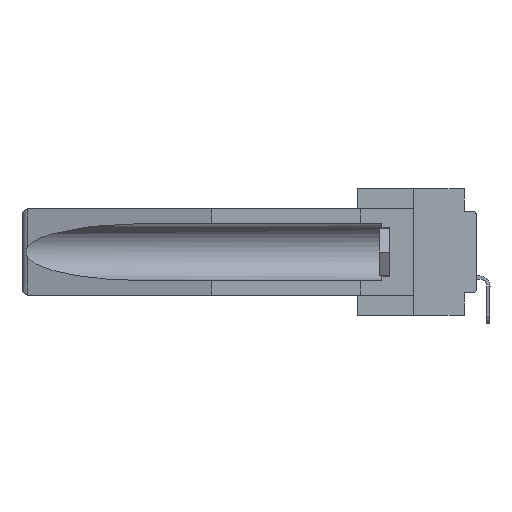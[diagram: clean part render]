
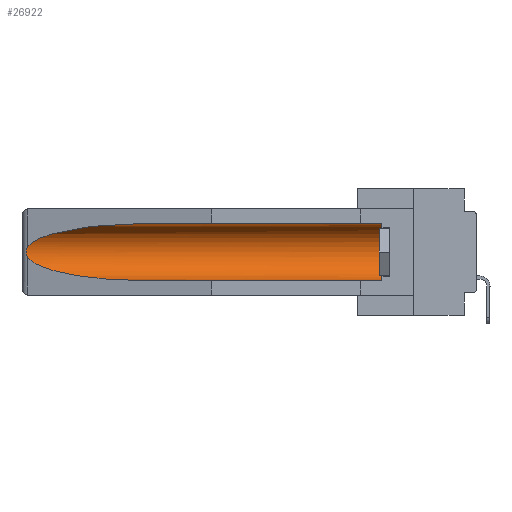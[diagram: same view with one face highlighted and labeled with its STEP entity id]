
A CAD part, left-side view. The second image highlights one B-rep face of the part: STEP entity #26922.
In plain terms, the highlighted cylindrical face has radius 2.857 mm (diameter 5.715 mm), a partial arc.
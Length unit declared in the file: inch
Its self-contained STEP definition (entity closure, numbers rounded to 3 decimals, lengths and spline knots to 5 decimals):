
#720 = DIRECTION ( 'NONE',  ( 0., 0., 1. ) ) ;
#1542 = EDGE_CURVE ( 'NONE', #3115, #8334, #3352, .T. ) ;
#2309 = ORIENTED_EDGE ( 'NONE', *, *, #4685, .T. ) ;
#2797 = EDGE_CURVE ( 'NONE', #3901, #11828, #21291, .T. ) ;
#2966 = CARTESIAN_POINT ( 'NONE',  ( 0.155, -0.30754, -0.1715 ) ) ;
#3114 = CARTESIAN_POINT ( 'NONE',  ( 0.2673, 1.5327, -0.16383 ) ) ;
#3115 = VERTEX_POINT ( 'NONE', #5909 ) ;
#3352 =( BOUNDED_CURVE ( )  B_SPLINE_CURVE ( 3, ( #6655, #21371, #31257, #21514 ),
 .UNSPECIFIED., .F., .T. ) 
 B_SPLINE_CURVE_WITH_KNOTS ( ( 4, 4 ),
 ( 4.71239, 6.08839 ),
 .UNSPECIFIED. ) 
 CURVE ( )  GEOMETRIC_REPRESENTATION_ITEM ( )  RATIONAL_B_SPLINE_CURVE ( ( 1., 0.848, 0.848, 1. ) ) 
 REPRESENTATION_ITEM ( '' )  );
#3901 = VERTEX_POINT ( 'NONE', #6263 ) ;
#4042 = ORIENTED_EDGE ( 'NONE', *, *, #2797, .F. ) ;
#4331 = CARTESIAN_POINT ( 'NONE',  ( 0.155, -0.30754, -0.284 ) ) ;
#4685 = EDGE_CURVE ( 'NONE', #8334, #18332, #13291, .T. ) ;
#4689 = VECTOR ( 'NONE', #21474, 39.37008 ) ;
#4727 = DIRECTION ( 'NONE',  ( 0., 0., 1. ) ) ;
#4944 = EDGE_CURVE ( 'NONE', #3901, #30158, #30249, .T. ) ;
#5623 = CARTESIAN_POINT ( 'NONE',  ( 0.155, 1.07973, -0.284 ) ) ;
#5909 = CARTESIAN_POINT ( 'NONE',  ( 0.155, 1.07973, -0.059 ) ) ;
#6025 = CARTESIAN_POINT ( 'NONE',  ( 0.2673, 1.53269, -0.17917 ) ) ;
#6038 = FACE_OUTER_BOUND ( 'NONE', #9230, .T. ) ;
#6116 = CARTESIAN_POINT ( 'NONE',  ( 0.21114, 1.30732, -0.284 ) ) ;
#6263 = CARTESIAN_POINT ( 'NONE',  ( 0.155, 0.126, -0.284 ) ) ;
#6655 = CARTESIAN_POINT ( 'NONE',  ( 0.155, 1.07973, -0.059 ) ) ;
#6661 = ORIENTED_EDGE ( 'NONE', *, *, #18236, .T. ) ;
#6783 = LINE ( 'NONE', #21328, #4689 ) ;
#8304 = CARTESIAN_POINT ( 'NONE',  ( 0.26655, 1.53094, -0.18657 ) ) ;
#8334 = VERTEX_POINT ( 'NONE', #29628 ) ;
#9230 = EDGE_LOOP ( 'NONE', ( #31022, #2309, #22160, #4042, #15883, #6661 ) ) ;
#10874 = CARTESIAN_POINT ( 'NONE',  ( 0.26597, 1.5296, -0.19026 ) ) ;
#11828 = VERTEX_POINT ( 'NONE', #5623 ) ;
#11921 = DIRECTION ( 'NONE',  ( 0., 1., 0. ) ) ;
#12840 = CARTESIAN_POINT ( 'NONE',  ( 0.26537, 1.52718, -0.14972 ) ) ;
#13243 = DIRECTION ( 'NONE',  ( 0., -1., 0. ) ) ;
#13280 =( BOUNDED_CURVE ( )  B_SPLINE_CURVE ( 3, ( #14213, #24045, #6116, #24677 ),
 .UNSPECIFIED., .F., .T. ) 
 B_SPLINE_CURVE_WITH_KNOTS ( ( 4, 4 ),
 ( 0.1948, 1.5708 ),
 .UNSPECIFIED. ) 
 CURVE ( )  GEOMETRIC_REPRESENTATION_ITEM ( )  RATIONAL_B_SPLINE_CURVE ( ( 1., 0.848, 0.848, 1. ) ) 
 REPRESENTATION_ITEM ( '' )  );
#13291 = B_SPLINE_CURVE_WITH_KNOTS ( 'NONE', 3,
 ( #12840, #20267, #30169, #3114, #28190, #20566, #6025, #8304, #10874, #18153 ),
 .UNSPECIFIED., .F., .F.,
 ( 4, 2, 2, 2, 4 ),
 ( 0., 0.00029, 0.00058, 0.00087, 0.00117 ),
 .UNSPECIFIED. ) ;
#13492 = DIRECTION ( 'NONE',  ( 0., 1., 0. ) ) ;
#14213 = CARTESIAN_POINT ( 'NONE',  ( 0.26537, 1.52718, -0.19328 ) ) ;
#15883 = ORIENTED_EDGE ( 'NONE', *, *, #4944, .T. ) ;
#16520 = CARTESIAN_POINT ( 'NONE',  ( 0.155, 0.126, -0.1715 ) ) ;
#17370 = VECTOR ( 'NONE', #11921, 39.37008 ) ;
#18153 = CARTESIAN_POINT ( 'NONE',  ( 0.26537, 1.52718, -0.19328 ) ) ;
#18236 = EDGE_CURVE ( 'NONE', #30158, #3115, #6783, .T. ) ;
#18332 = VERTEX_POINT ( 'NONE', #22102 ) ;
#20267 = CARTESIAN_POINT ( 'NONE',  ( 0.26597, 1.52961, -0.15275 ) ) ;
#20566 = CARTESIAN_POINT ( 'NONE',  ( 0.2675, 1.53308, -0.17534 ) ) ;
#21020 = EDGE_CURVE ( 'NONE', #18332, #11828, #13280, .T. ) ;
#21291 = LINE ( 'NONE', #4331, #17370 ) ;
#21328 = CARTESIAN_POINT ( 'NONE',  ( 0.155, -0.30754, -0.059 ) ) ;
#21371 = CARTESIAN_POINT ( 'NONE',  ( 0.21114, 1.30732, -0.059 ) ) ;
#21474 = DIRECTION ( 'NONE',  ( 0., 1., 0. ) ) ;
#21514 = CARTESIAN_POINT ( 'NONE',  ( 0.26537, 1.52718, -0.14972 ) ) ;
#22102 = CARTESIAN_POINT ( 'NONE',  ( 0.26537, 1.52718, -0.19328 ) ) ;
#22160 = ORIENTED_EDGE ( 'NONE', *, *, #21020, .T. ) ;
#24045 = CARTESIAN_POINT ( 'NONE',  ( 0.25451, 1.48313, -0.24835 ) ) ;
#24677 = CARTESIAN_POINT ( 'NONE',  ( 0.155, 1.07973, -0.284 ) ) ;
#25073 = CARTESIAN_POINT ( 'NONE',  ( 0.155, 0.126, -0.059 ) ) ;
#26922 = ADVANCED_FACE ( 'NONE', ( #6038 ), #30180, .F. ) ;
#28190 = CARTESIAN_POINT ( 'NONE',  ( 0.2675, 1.53308, -0.16763 ) ) ;
#29128 = AXIS2_PLACEMENT_3D ( 'NONE', #2966, #13492, #720 ) ;
#29628 = CARTESIAN_POINT ( 'NONE',  ( 0.26537, 1.52718, -0.14972 ) ) ;
#30158 = VERTEX_POINT ( 'NONE', #25073 ) ;
#30169 = CARTESIAN_POINT ( 'NONE',  ( 0.26654, 1.53092, -0.15636 ) ) ;
#30180 = CYLINDRICAL_SURFACE ( 'NONE', #29128, 0.1125 ) ;
#30249 = CIRCLE ( 'NONE', #31287, 0.1125 ) ;
#31022 = ORIENTED_EDGE ( 'NONE', *, *, #1542, .T. ) ;
#31257 = CARTESIAN_POINT ( 'NONE',  ( 0.25451, 1.48313, -0.09465 ) ) ;
#31287 = AXIS2_PLACEMENT_3D ( 'NONE', #16520, #13243, #4727 ) ;
